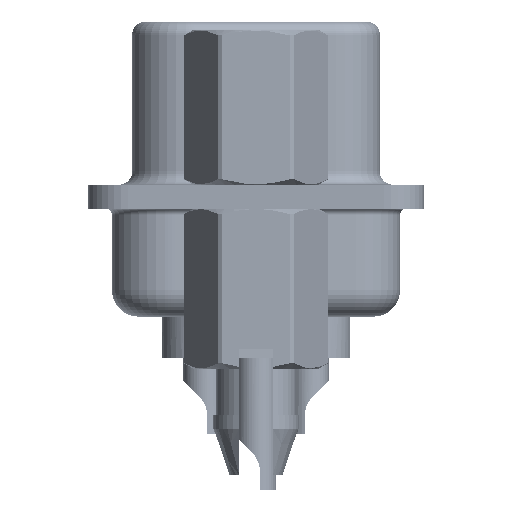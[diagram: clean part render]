
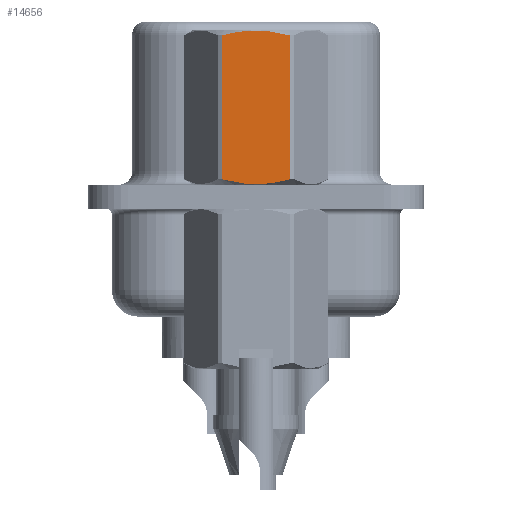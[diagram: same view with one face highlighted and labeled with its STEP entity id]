
A CAD part, left-side view. The second image highlights one B-rep face of the part: STEP entity #14656.
In plain terms, the highlighted planar face has unit normal (-1, 0, 0).
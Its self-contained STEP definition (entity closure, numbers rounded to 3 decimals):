
#335 = B_SPLINE_CURVE_WITH_KNOTS ( 'NONE', 3,
 ( #25577, #3821, #12104, #28442, #14655, #3645, #20576, #23088, #22904, #33463 ),
 .UNSPECIFIED., .F., .F.,
 ( 4, 2, 2, 2, 4 ),
 ( 0.001, 0.002, 0.002, 0.003, 0.004 ),
 .UNSPECIFIED. ) ;
#1769 = DIRECTION ( 'NONE',  ( -1., 0., 0. ) ) ;
#1963 = VERTEX_POINT ( 'NONE', #23233 ) ;
#2920 = EDGE_CURVE ( 'NONE', #6411, #1963, #11729, .T. ) ;
#3645 = CARTESIAN_POINT ( 'NONE',  ( -2.381, 0.215, 6.232 ) ) ;
#3821 = CARTESIAN_POINT ( 'NONE',  ( -2.381, -1.066, 6.104 ) ) ;
#5364 = CARTESIAN_POINT ( 'NONE',  ( -2.381, -0.215, 0.468 ) ) ;
#5537 = CARTESIAN_POINT ( 'NONE',  ( -2.381, -1.066, 0.596 ) ) ;
#6411 = VERTEX_POINT ( 'NONE', #16633 ) ;
#8226 = CARTESIAN_POINT ( 'NONE',  ( -2.381, 0.215, 0.468 ) ) ;
#8304 = AXIS2_PLACEMENT_3D ( 'NONE', #35187, #1769, #12583 ) ;
#9330 = VECTOR ( 'NONE', #26305, 1000. ) ;
#9427 = ORIENTED_EDGE ( 'NONE', *, *, #30863, .T. ) ;
#9852 = ORIENTED_EDGE ( 'NONE', *, *, #12063, .T. ) ;
#11101 = ORIENTED_EDGE ( 'NONE', *, *, #2920, .T. ) ;
#11512 = CARTESIAN_POINT ( 'NONE',  ( -2.381, -1.273, 6.048 ) ) ;
#11729 = LINE ( 'NONE', #12263, #26281 ) ;
#11853 = VERTEX_POINT ( 'NONE', #12129 ) ;
#12063 = EDGE_CURVE ( 'NONE', #11853, #28112, #15394, .T. ) ;
#12104 = CARTESIAN_POINT ( 'NONE',  ( -2.381, -0.858, 6.15 ) ) ;
#12129 = CARTESIAN_POINT ( 'NONE',  ( -2.381, -1.273, 0.652 ) ) ;
#12263 = CARTESIAN_POINT ( 'NONE',  ( -2.381, 1.273, 3.792 ) ) ;
#12583 = DIRECTION ( 'NONE',  ( 0., -1., 0. ) ) ;
#13670 = CARTESIAN_POINT ( 'NONE',  ( -2.381, -0.432, 0.485 ) ) ;
#14655 = CARTESIAN_POINT ( 'NONE',  ( -2.381, -0.215, 6.232 ) ) ;
#14656 = ADVANCED_FACE ( 'NONE', ( #20886 ), #26943, .T. ) ;
#15394 = LINE ( 'NONE', #35093, #9330 ) ;
#15855 = CARTESIAN_POINT ( 'NONE',  ( -2.381, -0.858, 0.55 ) ) ;
#16633 = CARTESIAN_POINT ( 'NONE',  ( -2.381, 1.273, 6.048 ) ) ;
#17180 = EDGE_LOOP ( 'NONE', ( #9427, #9852, #20246, #11101 ) ) ;
#19078 = CARTESIAN_POINT ( 'NONE',  ( -2.381, 0.853, 0.549 ) ) ;
#20246 = ORIENTED_EDGE ( 'NONE', *, *, #24043, .T. ) ;
#20576 = CARTESIAN_POINT ( 'NONE',  ( -2.381, 0.428, 6.215 ) ) ;
#20886 = FACE_OUTER_BOUND ( 'NONE', #17180, .T. ) ;
#21767 = CARTESIAN_POINT ( 'NONE',  ( -2.381, 1.065, 0.596 ) ) ;
#21835 = B_SPLINE_CURVE_WITH_KNOTS ( 'NONE', 3,
 ( #35375, #21767, #19078, #29992, #8226, #5364, #13670, #15855, #5537, #26603 ),
 .UNSPECIFIED., .F., .F.,
 ( 4, 2, 2, 2, 4 ),
 ( 0.003, 0.003, 0.004, 0.004, 0.005 ),
 .UNSPECIFIED. ) ;
#22904 = CARTESIAN_POINT ( 'NONE',  ( -2.381, 1.065, 6.104 ) ) ;
#23088 = CARTESIAN_POINT ( 'NONE',  ( -2.381, 0.853, 6.151 ) ) ;
#23233 = CARTESIAN_POINT ( 'NONE',  ( -2.381, 1.273, 0.652 ) ) ;
#24043 = EDGE_CURVE ( 'NONE', #28112, #6411, #335, .T. ) ;
#25577 = CARTESIAN_POINT ( 'NONE',  ( -2.381, -1.273, 6.048 ) ) ;
#26281 = VECTOR ( 'NONE', #33793, 1000. ) ;
#26305 = DIRECTION ( 'NONE',  ( 0., 0., 1. ) ) ;
#26603 = CARTESIAN_POINT ( 'NONE',  ( -2.381, -1.273, 0.652 ) ) ;
#26943 = PLANE ( 'NONE',  #8304 ) ;
#28112 = VERTEX_POINT ( 'NONE', #11512 ) ;
#28442 = CARTESIAN_POINT ( 'NONE',  ( -2.381, -0.432, 6.215 ) ) ;
#29992 = CARTESIAN_POINT ( 'NONE',  ( -2.381, 0.428, 0.485 ) ) ;
#30863 = EDGE_CURVE ( 'NONE', #1963, #11853, #21835, .T. ) ;
#33463 = CARTESIAN_POINT ( 'NONE',  ( -2.381, 1.273, 6.048 ) ) ;
#33793 = DIRECTION ( 'NONE',  ( 0., 0., -1. ) ) ;
#35093 = CARTESIAN_POINT ( 'NONE',  ( -2.381, -1.273, 3.792 ) ) ;
#35187 = CARTESIAN_POINT ( 'NONE',  ( -2.381, 1.375, -3.75 ) ) ;
#35375 = CARTESIAN_POINT ( 'NONE',  ( -2.381, 1.273, 0.652 ) ) ;
